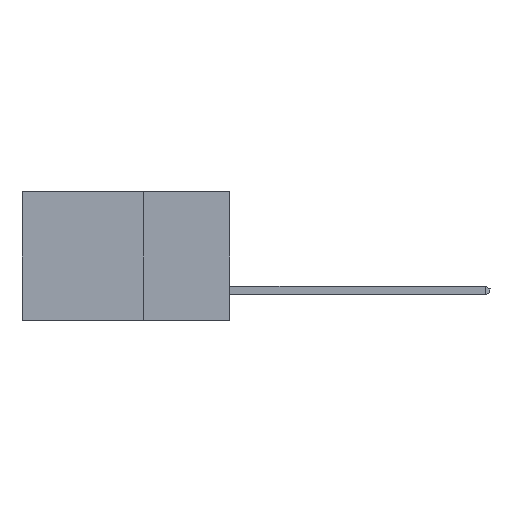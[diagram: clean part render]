
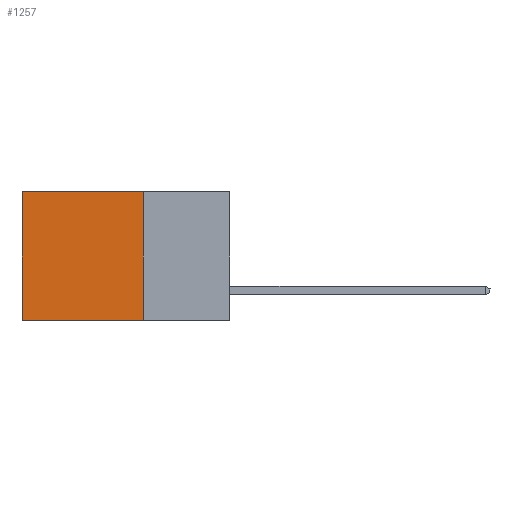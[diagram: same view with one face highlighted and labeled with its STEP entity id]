
A CAD part, left-side view. The second image highlights one B-rep face of the part: STEP entity #1257.
In plain terms, the highlighted planar face has unit normal (-1, 0, 0).
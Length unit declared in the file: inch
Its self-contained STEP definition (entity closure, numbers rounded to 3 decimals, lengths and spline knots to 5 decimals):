
#54 = CARTESIAN_POINT ( 'NONE',  ( 0.2615, 0.25, -0.37 ) ) ;
#581 = ORIENTED_EDGE ( 'NONE', *, *, #13398, .T. ) ;
#870 = VECTOR ( 'NONE', #6281, 39.37008 ) ;
#1257 = ADVANCED_FACE ( 'NONE', ( #17486 ), #1451, .F. ) ;
#1451 = PLANE ( 'NONE',  #6156 ) ;
#1548 = DIRECTION ( 'NONE',  ( 0., 0., -1. ) ) ;
#1818 = LINE ( 'NONE', #13944, #870 ) ;
#1822 = VERTEX_POINT ( 'NONE', #17904 ) ;
#2694 = VERTEX_POINT ( 'NONE', #9425 ) ;
#2852 = CARTESIAN_POINT ( 'NONE',  ( 0.2615, 0.6, -0.37 ) ) ;
#4203 = EDGE_CURVE ( 'NONE', #1822, #8729, #17468, .T. ) ;
#4300 = ORIENTED_EDGE ( 'NONE', *, *, #15923, .F. ) ;
#4520 = CARTESIAN_POINT ( 'NONE',  ( 0.2615, 0.6, -0.37 ) ) ;
#5451 = ORIENTED_EDGE ( 'NONE', *, *, #4203, .T. ) ;
#6156 = AXIS2_PLACEMENT_3D ( 'NONE', #7052, #12856, #1548 ) ;
#6281 = DIRECTION ( 'NONE',  ( 0., 1., 0. ) ) ;
#7052 = CARTESIAN_POINT ( 'NONE',  ( 0.2615, 0.25, -0.37 ) ) ;
#7584 = VECTOR ( 'NONE', #17460, 39.37008 ) ;
#8729 = VERTEX_POINT ( 'NONE', #4520 ) ;
#9425 = CARTESIAN_POINT ( 'NONE',  ( 0.2615, 0.25, -0.37 ) ) ;
#9811 = VECTOR ( 'NONE', #9980, 39.37008 ) ;
#9866 = EDGE_CURVE ( 'NONE', #2694, #8729, #1818, .T. ) ;
#9980 = DIRECTION ( 'NONE',  ( 0., 0., -1. ) ) ;
#10031 = DIRECTION ( 'NONE',  ( 0., 0., -1. ) ) ;
#10333 = ORIENTED_EDGE ( 'NONE', *, *, #9866, .F. ) ;
#11673 = CARTESIAN_POINT ( 'NONE',  ( 0.2615, 0.25, 0. ) ) ;
#11719 = EDGE_LOOP ( 'NONE', ( #5451, #10333, #4300, #581 ) ) ;
#12856 = DIRECTION ( 'NONE',  ( 1., 0., 0. ) ) ;
#13398 = EDGE_CURVE ( 'NONE', #17948, #1822, #17738, .T. ) ;
#13944 = CARTESIAN_POINT ( 'NONE',  ( 0.2615, 0.25, -0.37 ) ) ;
#15923 = EDGE_CURVE ( 'NONE', #17948, #2694, #17434, .T. ) ;
#16366 = CARTESIAN_POINT ( 'NONE',  ( 0.2615, 0.25, 0. ) ) ;
#17051 = VECTOR ( 'NONE', #10031, 39.37008 ) ;
#17434 = LINE ( 'NONE', #54, #17051 ) ;
#17460 = DIRECTION ( 'NONE',  ( 0., 1., 0. ) ) ;
#17468 = LINE ( 'NONE', #2852, #9811 ) ;
#17486 = FACE_OUTER_BOUND ( 'NONE', #11719, .T. ) ;
#17738 = LINE ( 'NONE', #11673, #7584 ) ;
#17904 = CARTESIAN_POINT ( 'NONE',  ( 0.2615, 0.6, 0. ) ) ;
#17948 = VERTEX_POINT ( 'NONE', #16366 ) ;
